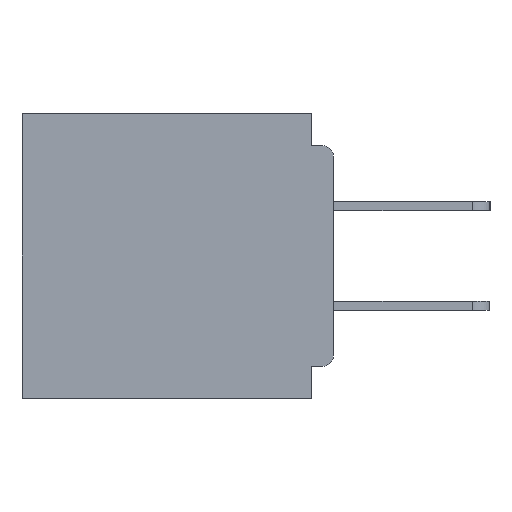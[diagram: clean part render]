
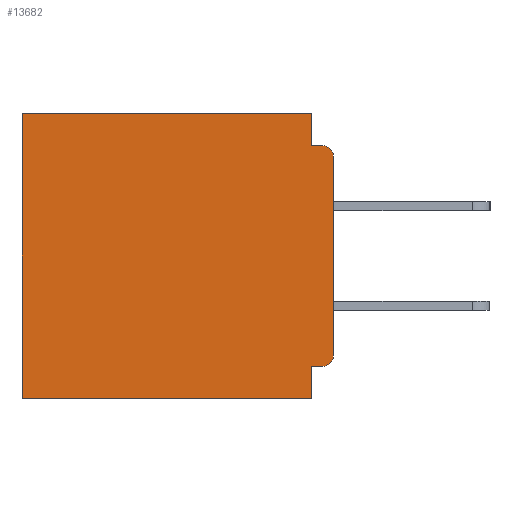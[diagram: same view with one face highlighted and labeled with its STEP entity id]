
A CAD part, left-side view. The second image highlights one B-rep face of the part: STEP entity #13682.
In plain terms, the highlighted planar face has unit normal (-1, 0, 0).
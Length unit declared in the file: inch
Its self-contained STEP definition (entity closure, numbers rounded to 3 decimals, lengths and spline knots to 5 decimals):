
#72 = CIRCLE ( 'NONE', #34281, 0.015 ) ;
#428 = LINE ( 'NONE', #12710, #29782 ) ;
#1376 = VERTEX_POINT ( 'NONE', #24684 ) ;
#1491 = FACE_OUTER_BOUND ( 'NONE', #21288, .T. ) ;
#2532 = VECTOR ( 'NONE', #25428, 39.37008 ) ;
#3305 = CARTESIAN_POINT ( 'NONE',  ( 0.3, 0., 0. ) ) ;
#3724 = CARTESIAN_POINT ( 'NONE',  ( 0.3, 0., -0.06 ) ) ;
#4746 = CARTESIAN_POINT ( 'NONE',  ( 0.3, 0., -0.34 ) ) ;
#4830 = LINE ( 'NONE', #5261, #26642 ) ;
#5118 = CARTESIAN_POINT ( 'NONE',  ( 0.3, 0.015, -0.355 ) ) ;
#5261 = CARTESIAN_POINT ( 'NONE',  ( 0.3, 0., -0.4 ) ) ;
#5589 = VECTOR ( 'NONE', #6193, 39.37008 ) ;
#5866 = LINE ( 'NONE', #17412, #34077 ) ;
#6193 = DIRECTION ( 'NONE',  ( 0., 1., 0. ) ) ;
#7368 = VECTOR ( 'NONE', #34039, 39.37008 ) ;
#7580 = PLANE ( 'NONE',  #23021 ) ;
#7666 = VERTEX_POINT ( 'NONE', #14555 ) ;
#8683 = ORIENTED_EDGE ( 'NONE', *, *, #24529, .F. ) ;
#9001 = DIRECTION ( 'NONE',  ( -1., 0., 0. ) ) ;
#9077 = EDGE_CURVE ( 'NONE', #36001, #24408, #5866, .T. ) ;
#10522 = CARTESIAN_POINT ( 'NONE',  ( 0.3, 0., -0.4 ) ) ;
#10545 = ORIENTED_EDGE ( 'NONE', *, *, #11988, .T. ) ;
#11116 = DIRECTION ( 'NONE',  ( 0., 0., -1. ) ) ;
#11141 = LINE ( 'NONE', #36357, #2532 ) ;
#11988 = EDGE_CURVE ( 'NONE', #32337, #1376, #13754, .T. ) ;
#12710 = CARTESIAN_POINT ( 'NONE',  ( 0.3, 0., -0.045 ) ) ;
#12906 = DIRECTION ( 'NONE',  ( 0., 0., -1. ) ) ;
#13266 = LINE ( 'NONE', #23227, #5589 ) ;
#13412 = DIRECTION ( 'NONE',  ( 0., 0., -1. ) ) ;
#13682 = ADVANCED_FACE ( 'NONE', ( #1491 ), #7580, .F. ) ;
#13754 = CIRCLE ( 'NONE', #23454, 0.015 ) ;
#13813 = VECTOR ( 'NONE', #34411, 39.37008 ) ;
#14555 = CARTESIAN_POINT ( 'NONE',  ( 0.3, 0.031, -0.4 ) ) ;
#14780 = CARTESIAN_POINT ( 'NONE',  ( 0.3, 0.015, -0.06 ) ) ;
#16312 = ORIENTED_EDGE ( 'NONE', *, *, #21769, .F. ) ;
#16552 = EDGE_CURVE ( 'NONE', #17481, #36001, #29647, .T. ) ;
#17412 = CARTESIAN_POINT ( 'NONE',  ( 0.3, 0.437, -0.4 ) ) ;
#17481 = VERTEX_POINT ( 'NONE', #32789 ) ;
#17583 = DIRECTION ( 'NONE',  ( 0., 0., -1. ) ) ;
#19290 = CARTESIAN_POINT ( 'NONE',  ( 0.3, 0.437, 0. ) ) ;
#19669 = CARTESIAN_POINT ( 'NONE',  ( 0.3, 0.437, -0.4 ) ) ;
#20303 = EDGE_CURVE ( 'NONE', #31363, #1376, #428, .T. ) ;
#21288 = EDGE_LOOP ( 'NONE', ( #16312, #10545, #30559, #32936, #35636, #27967, #26139, #33484, #8683, #25840 ) ) ;
#21769 = EDGE_CURVE ( 'NONE', #32337, #29026, #4830, .T. ) ;
#21970 = CARTESIAN_POINT ( 'NONE',  ( 0.3, 0.031, -0.045 ) ) ;
#22985 = CARTESIAN_POINT ( 'NONE',  ( 0.3, 0., -0.355 ) ) ;
#23021 = AXIS2_PLACEMENT_3D ( 'NONE', #10522, #30227, #13412 ) ;
#23227 = CARTESIAN_POINT ( 'NONE',  ( 0.3, 0., -0.4 ) ) ;
#23454 = AXIS2_PLACEMENT_3D ( 'NONE', #14780, #34272, #17583 ) ;
#24408 = VERTEX_POINT ( 'NONE', #19669 ) ;
#24529 = EDGE_CURVE ( 'NONE', #29090, #36181, #31706, .T. ) ;
#24569 = EDGE_CURVE ( 'NONE', #7666, #24408, #13266, .T. ) ;
#24684 = CARTESIAN_POINT ( 'NONE',  ( 0.3, 0.015, -0.045 ) ) ;
#25428 = DIRECTION ( 'NONE',  ( 0., 0., -1. ) ) ;
#25840 = ORIENTED_EDGE ( 'NONE', *, *, #28152, .T. ) ;
#25903 = DIRECTION ( 'NONE',  ( 0., 0., -1. ) ) ;
#25959 = CARTESIAN_POINT ( 'NONE',  ( 0.3, 0.015, -0.34 ) ) ;
#26139 = ORIENTED_EDGE ( 'NONE', *, *, #24569, .F. ) ;
#26642 = VECTOR ( 'NONE', #11116, 39.37008 ) ;
#27967 = ORIENTED_EDGE ( 'NONE', *, *, #9077, .T. ) ;
#28152 = EDGE_CURVE ( 'NONE', #29090, #29026, #72, .T. ) ;
#28375 = EDGE_CURVE ( 'NONE', #17481, #31363, #36251, .T. ) ;
#28793 = DIRECTION ( 'NONE',  ( 0., 0., -1. ) ) ;
#29026 = VERTEX_POINT ( 'NONE', #4746 ) ;
#29036 = VECTOR ( 'NONE', #12906, 39.37008 ) ;
#29090 = VERTEX_POINT ( 'NONE', #5118 ) ;
#29544 = DIRECTION ( 'NONE',  ( 0., -1., 0. ) ) ;
#29647 = LINE ( 'NONE', #3305, #13813 ) ;
#29782 = VECTOR ( 'NONE', #29544, 39.37008 ) ;
#30227 = DIRECTION ( 'NONE',  ( 1., 0., 0. ) ) ;
#30559 = ORIENTED_EDGE ( 'NONE', *, *, #20303, .F. ) ;
#31363 = VERTEX_POINT ( 'NONE', #21970 ) ;
#31706 = LINE ( 'NONE', #22985, #7368 ) ;
#32337 = VERTEX_POINT ( 'NONE', #3724 ) ;
#32373 = CARTESIAN_POINT ( 'NONE',  ( 0.3, 0.031, 0. ) ) ;
#32789 = CARTESIAN_POINT ( 'NONE',  ( 0.3, 0.031, 0. ) ) ;
#32936 = ORIENTED_EDGE ( 'NONE', *, *, #28375, .F. ) ;
#33484 = ORIENTED_EDGE ( 'NONE', *, *, #34916, .F. ) ;
#33905 = CARTESIAN_POINT ( 'NONE',  ( 0.3, 0.031, -0.355 ) ) ;
#34039 = DIRECTION ( 'NONE',  ( 0., 1., 0. ) ) ;
#34077 = VECTOR ( 'NONE', #25903, 39.37008 ) ;
#34272 = DIRECTION ( 'NONE',  ( -1., 0., 0. ) ) ;
#34281 = AXIS2_PLACEMENT_3D ( 'NONE', #25959, #9001, #28793 ) ;
#34411 = DIRECTION ( 'NONE',  ( 0., 1., 0. ) ) ;
#34916 = EDGE_CURVE ( 'NONE', #36181, #7666, #11141, .T. ) ;
#35636 = ORIENTED_EDGE ( 'NONE', *, *, #16552, .T. ) ;
#36001 = VERTEX_POINT ( 'NONE', #19290 ) ;
#36181 = VERTEX_POINT ( 'NONE', #33905 ) ;
#36251 = LINE ( 'NONE', #32373, #29036 ) ;
#36357 = CARTESIAN_POINT ( 'NONE',  ( 0.3, 0.031, -0.4 ) ) ;
